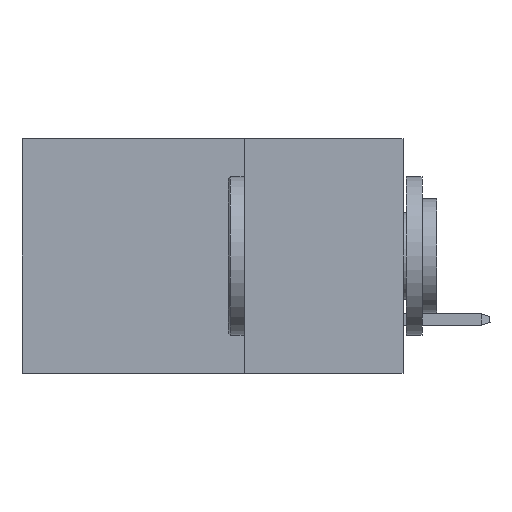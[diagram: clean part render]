
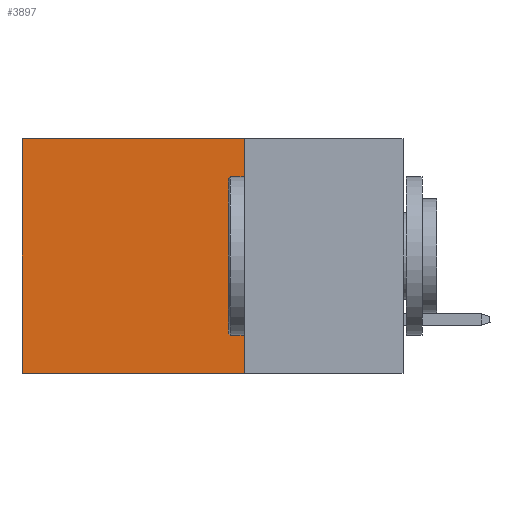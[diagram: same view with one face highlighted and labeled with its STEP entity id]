
A CAD part, left-side view. The second image highlights one B-rep face of the part: STEP entity #3897.
In plain terms, the highlighted planar face has unit normal (-1, 0, 0).
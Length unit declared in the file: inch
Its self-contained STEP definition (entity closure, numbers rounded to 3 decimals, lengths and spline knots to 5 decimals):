
#607 = LINE ( 'NONE', #18456, #6961 ) ;
#3897 = ADVANCED_FACE ( 'NONE', ( #16219 ), #4183, .F. ) ;
#3992 = LINE ( 'NONE', #16020, #7472 ) ;
#4183 = PLANE ( 'NONE',  #12625 ) ;
#4192 = LINE ( 'NONE', #23981, #7245 ) ;
#4387 = CARTESIAN_POINT ( 'NONE',  ( 0.2875, 0.6, -0.37 ) ) ;
#4557 = ORIENTED_EDGE ( 'NONE', *, *, #8576, .T. ) ;
#4563 = LINE ( 'NONE', #20479, #19848 ) ;
#6961 = VECTOR ( 'NONE', #14566, 39.37008 ) ;
#7245 = VECTOR ( 'NONE', #11843, 39.37008 ) ;
#7472 = VECTOR ( 'NONE', #20293, 39.37008 ) ;
#8006 = VERTEX_POINT ( 'NONE', #4387 ) ;
#8096 = ORIENTED_EDGE ( 'NONE', *, *, #22596, .F. ) ;
#8576 = EDGE_CURVE ( 'NONE', #16665, #21610, #607, .T. ) ;
#10147 = EDGE_CURVE ( 'NONE', #21610, #8006, #4192, .T. ) ;
#11843 = DIRECTION ( 'NONE',  ( 0., 0., -1. ) ) ;
#12218 = CARTESIAN_POINT ( 'NONE',  ( 0.2875, 0.25, 0. ) ) ;
#12625 = AXIS2_PLACEMENT_3D ( 'NONE', #12218, #14273, #18164 ) ;
#12698 = ORIENTED_EDGE ( 'NONE', *, *, #10147, .T. ) ;
#14273 = DIRECTION ( 'NONE',  ( 1., 0., 0. ) ) ;
#14566 = DIRECTION ( 'NONE',  ( 0., 1., 0. ) ) ;
#14727 = VERTEX_POINT ( 'NONE', #22148 ) ;
#16020 = CARTESIAN_POINT ( 'NONE',  ( 0.2875, 0.25, 0. ) ) ;
#16219 = FACE_OUTER_BOUND ( 'NONE', #25505, .T. ) ;
#16665 = VERTEX_POINT ( 'NONE', #22750 ) ;
#17455 = EDGE_CURVE ( 'NONE', #16665, #14727, #3992, .T. ) ;
#18164 = DIRECTION ( 'NONE',  ( 0., 0., -1. ) ) ;
#18456 = CARTESIAN_POINT ( 'NONE',  ( 0.2875, 0.25, 0. ) ) ;
#19848 = VECTOR ( 'NONE', #22396, 39.37008 ) ;
#20293 = DIRECTION ( 'NONE',  ( 0., 0., -1. ) ) ;
#20479 = CARTESIAN_POINT ( 'NONE',  ( 0.2875, 0.25, -0.37 ) ) ;
#20620 = ORIENTED_EDGE ( 'NONE', *, *, #17455, .F. ) ;
#21477 = CARTESIAN_POINT ( 'NONE',  ( 0.2875, 0.6, 0. ) ) ;
#21610 = VERTEX_POINT ( 'NONE', #21477 ) ;
#22148 = CARTESIAN_POINT ( 'NONE',  ( 0.2875, 0.25, -0.37 ) ) ;
#22396 = DIRECTION ( 'NONE',  ( 0., 1., 0. ) ) ;
#22596 = EDGE_CURVE ( 'NONE', #14727, #8006, #4563, .T. ) ;
#22750 = CARTESIAN_POINT ( 'NONE',  ( 0.2875, 0.25, 0. ) ) ;
#23981 = CARTESIAN_POINT ( 'NONE',  ( 0.2875, 0.6, 0. ) ) ;
#25505 = EDGE_LOOP ( 'NONE', ( #12698, #8096, #20620, #4557 ) ) ;
